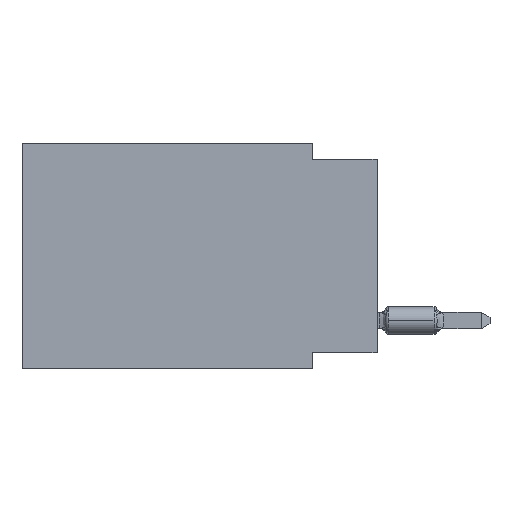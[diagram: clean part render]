
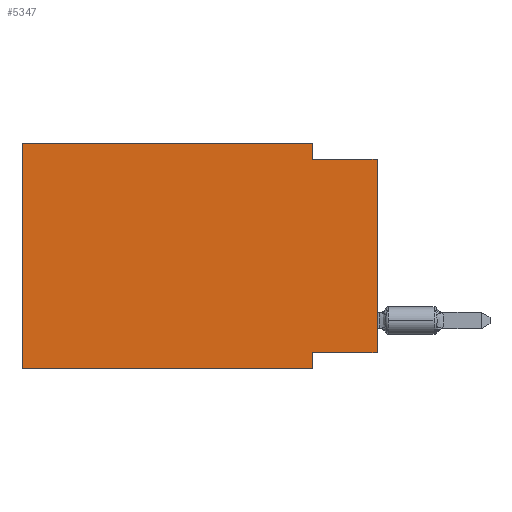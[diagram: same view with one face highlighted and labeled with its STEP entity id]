
A CAD part, left-side view. The second image highlights one B-rep face of the part: STEP entity #5347.
In plain terms, the highlighted planar face has unit normal (-1, 0, 0).
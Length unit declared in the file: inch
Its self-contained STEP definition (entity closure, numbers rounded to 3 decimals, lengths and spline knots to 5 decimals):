
#57 = ORIENTED_EDGE ( 'NONE', *, *, #12785, .T. ) ;
#165 = VECTOR ( 'NONE', #1895, 39.37008 ) ;
#215 = EDGE_LOOP ( 'NONE', ( #57, #2514, #11674, #2634, #3468, #5116, #912, #2976 ) ) ;
#278 = EDGE_CURVE ( 'NONE', #11522, #13070, #11005, .T. ) ;
#350 = EDGE_CURVE ( 'NONE', #12158, #13125, #12745, .T. ) ;
#858 = CARTESIAN_POINT ( 'NONE',  ( 0., 0., -0.025 ) ) ;
#912 = ORIENTED_EDGE ( 'NONE', *, *, #9786, .F. ) ;
#1185 = VECTOR ( 'NONE', #9587, 39.37008 ) ;
#1424 = CARTESIAN_POINT ( 'NONE',  ( 0., 0.55, 0. ) ) ;
#1656 = CARTESIAN_POINT ( 'NONE',  ( 0., 0.55, -0.35 ) ) ;
#1895 = DIRECTION ( 'NONE',  ( 0., -1., 0. ) ) ;
#1903 = CARTESIAN_POINT ( 'NONE',  ( 0., 0.55, 0. ) ) ;
#2216 = VECTOR ( 'NONE', #6526, 39.37008 ) ;
#2514 = ORIENTED_EDGE ( 'NONE', *, *, #6809, .F. ) ;
#2617 = DIRECTION ( 'NONE',  ( 0., 0., 1. ) ) ;
#2634 = ORIENTED_EDGE ( 'NONE', *, *, #278, .F. ) ;
#2758 = PLANE ( 'NONE',  #11239 ) ;
#2976 = ORIENTED_EDGE ( 'NONE', *, *, #350, .F. ) ;
#2979 = CARTESIAN_POINT ( 'NONE',  ( 0., 0., -0.325 ) ) ;
#3223 = CARTESIAN_POINT ( 'NONE',  ( 0., 0.55, -0.35 ) ) ;
#3243 = LINE ( 'NONE', #858, #165 ) ;
#3468 = ORIENTED_EDGE ( 'NONE', *, *, #8107, .F. ) ;
#3676 = CARTESIAN_POINT ( 'NONE',  ( 0., 0., -0.325 ) ) ;
#3822 = CARTESIAN_POINT ( 'NONE',  ( 0., 0.55, 0. ) ) ;
#4555 = LINE ( 'NONE', #3223, #10008 ) ;
#4852 = DIRECTION ( 'NONE',  ( 1., 0., 0. ) ) ;
#5116 = ORIENTED_EDGE ( 'NONE', *, *, #11053, .T. ) ;
#5216 = VERTEX_POINT ( 'NONE', #10675 ) ;
#5293 = CARTESIAN_POINT ( 'NONE',  ( 0., 0.1, -0.35 ) ) ;
#5347 = ADVANCED_FACE ( 'NONE', ( #11274 ), #2758, .F. ) ;
#5577 = VECTOR ( 'NONE', #6654, 39.37008 ) ;
#6109 = VERTEX_POINT ( 'NONE', #11346 ) ;
#6248 = DIRECTION ( 'NONE',  ( 0., 0., -1. ) ) ;
#6526 = DIRECTION ( 'NONE',  ( 0., 0., 1. ) ) ;
#6654 = DIRECTION ( 'NONE',  ( 0., -1., 0. ) ) ;
#6719 = LINE ( 'NONE', #8572, #1185 ) ;
#6809 = EDGE_CURVE ( 'NONE', #5216, #6109, #3243, .T. ) ;
#7317 = VECTOR ( 'NONE', #2617, 39.37008 ) ;
#7353 = VECTOR ( 'NONE', #9800, 39.37008 ) ;
#7640 = LINE ( 'NONE', #10825, #7317 ) ;
#8107 = EDGE_CURVE ( 'NONE', #13027, #11522, #7640, .T. ) ;
#8232 = VECTOR ( 'NONE', #6248, 39.37008 ) ;
#8371 = VERTEX_POINT ( 'NONE', #5293 ) ;
#8572 = CARTESIAN_POINT ( 'NONE',  ( 0., 0.1, -0.35 ) ) ;
#9386 = CARTESIAN_POINT ( 'NONE',  ( 0., 0.1, 0. ) ) ;
#9587 = DIRECTION ( 'NONE',  ( 0., 0., -1. ) ) ;
#9786 = EDGE_CURVE ( 'NONE', #13125, #8371, #6719, .T. ) ;
#9800 = DIRECTION ( 'NONE',  ( 0., 1., 0. ) ) ;
#10008 = VECTOR ( 'NONE', #10380, 39.37008 ) ;
#10380 = DIRECTION ( 'NONE',  ( 0., -1., 0. ) ) ;
#10675 = CARTESIAN_POINT ( 'NONE',  ( 0., 0.1, -0.025 ) ) ;
#10825 = CARTESIAN_POINT ( 'NONE',  ( 0., 0.55, 0. ) ) ;
#11005 = LINE ( 'NONE', #1424, #5577 ) ;
#11053 = EDGE_CURVE ( 'NONE', #13027, #8371, #4555, .T. ) ;
#11239 = AXIS2_PLACEMENT_3D ( 'NONE', #3822, #4852, #11994 ) ;
#11274 = FACE_OUTER_BOUND ( 'NONE', #215, .T. ) ;
#11346 = CARTESIAN_POINT ( 'NONE',  ( 0., 0., -0.025 ) ) ;
#11522 = VERTEX_POINT ( 'NONE', #1903 ) ;
#11674 = ORIENTED_EDGE ( 'NONE', *, *, #12251, .F. ) ;
#11994 = DIRECTION ( 'NONE',  ( 0., 0., -1. ) ) ;
#12158 = VERTEX_POINT ( 'NONE', #2979 ) ;
#12165 = CARTESIAN_POINT ( 'NONE',  ( 0., 0.1, -0.325 ) ) ;
#12251 = EDGE_CURVE ( 'NONE', #13070, #5216, #13307, .T. ) ;
#12487 = LINE ( 'NONE', #12603, #2216 ) ;
#12603 = CARTESIAN_POINT ( 'NONE',  ( 0., 0., 0. ) ) ;
#12745 = LINE ( 'NONE', #3676, #7353 ) ;
#12785 = EDGE_CURVE ( 'NONE', #12158, #6109, #12487, .T. ) ;
#13027 = VERTEX_POINT ( 'NONE', #1656 ) ;
#13057 = CARTESIAN_POINT ( 'NONE',  ( 0., 0.1, 0. ) ) ;
#13070 = VERTEX_POINT ( 'NONE', #13057 ) ;
#13125 = VERTEX_POINT ( 'NONE', #12165 ) ;
#13307 = LINE ( 'NONE', #9386, #8232 ) ;
